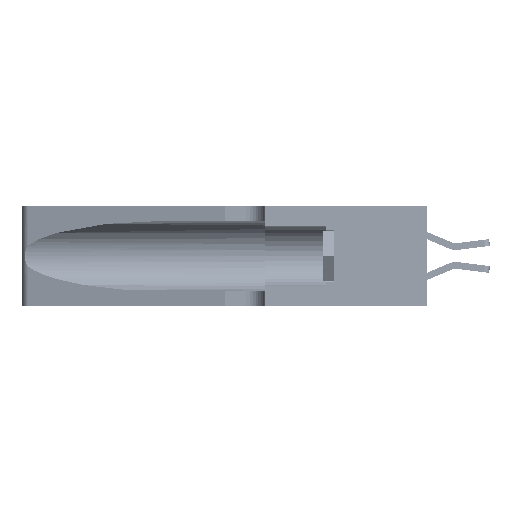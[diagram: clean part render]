
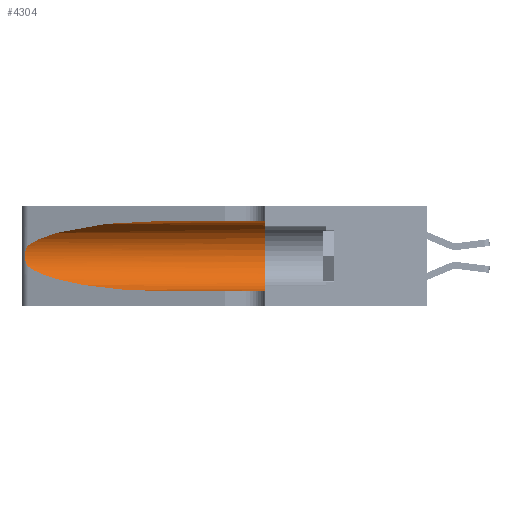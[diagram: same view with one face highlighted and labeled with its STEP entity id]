
A CAD part, left-side view. The second image highlights one B-rep face of the part: STEP entity #4304.
In plain terms, the highlighted cylindrical face has radius 3.308 mm (diameter 6.617 mm), a partial arc.
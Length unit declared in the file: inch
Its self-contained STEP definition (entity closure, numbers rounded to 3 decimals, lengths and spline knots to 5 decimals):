
#929 = ORIENTED_EDGE ( 'NONE', *, *, #17783, .T. ) ;
#1573 = B_SPLINE_CURVE_WITH_KNOTS ( 'NONE', 3,
 ( #2496, #9038, #37356, #37505, #5739, #18394, #12480, #27633, #30977, #40392, #37071, #21547, #21409, #21273 ),
 .UNSPECIFIED., .F., .F.,
 ( 4, 2, 2, 2, 2, 2, 4 ),
 ( 0., 0.00027, 0.00053, 0.00107, 0.0016, 0.00187, 0.00214 ),
 .UNSPECIFIED. ) ;
#1955 = CARTESIAN_POINT ( 'NONE',  ( 0.1305, 0.35, 0.31525 ) ) ;
#2175 = CARTESIAN_POINT ( 'NONE',  ( 0.1305, 0.35, 0.185 ) ) ;
#2311 = CARTESIAN_POINT ( 'NONE',  ( 0.1305, 1.61858, 0.05475 ) ) ;
#2496 = CARTESIAN_POINT ( 'NONE',  ( 0.25487, 1.22718, 0.22369 ) ) ;
#2839 = CARTESIAN_POINT ( 'NONE',  ( 0.25487, 1.22718, 0.22369 ) ) ;
#4304 = ADVANCED_FACE ( 'NONE', ( #5860 ), #30027, .F. ) ;
#5739 = CARTESIAN_POINT ( 'NONE',  ( 0.25854, 1.2359, 0.20912 ) ) ;
#5860 = FACE_OUTER_BOUND ( 'NONE', #28260, .T. ) ;
#6360 = CARTESIAN_POINT ( 'NONE',  ( 0.2373, 1.15595, 0.28018 ) ) ;
#6458 = EDGE_CURVE ( 'NONE', #25849, #38129, #1573, .T. ) ;
#6865 = VERTEX_POINT ( 'NONE', #19688 ) ;
#7002 =( BOUNDED_CURVE ( )  B_SPLINE_CURVE ( 3, ( #29686, #35947, #21110, #39104 ),
 .UNSPECIFIED., .F., .T. ) 
 B_SPLINE_CURVE_WITH_KNOTS ( ( 4, 4 ),
 ( 3.44316, 4.71239 ),
 .UNSPECIFIED. ) 
 CURVE ( )  GEOMETRIC_REPRESENTATION_ITEM ( )  RATIONAL_B_SPLINE_CURVE ( ( 1., 0.87, 0.87, 1. ) ) 
 REPRESENTATION_ITEM ( '' )  );
#7755 = ORIENTED_EDGE ( 'NONE', *, *, #6458, .T. ) ;
#8426 = DIRECTION ( 'NONE',  ( 0., 0., 1. ) ) ;
#8849 = ORIENTED_EDGE ( 'NONE', *, *, #15151, .F. ) ;
#9038 = CARTESIAN_POINT ( 'NONE',  ( 0.25555, 1.22994, 0.2215 ) ) ;
#9274 = ORIENTED_EDGE ( 'NONE', *, *, #15804, .T. ) ;
#9495 = CARTESIAN_POINT ( 'NONE',  ( 0.25487, 1.22718, 0.22369 ) ) ;
#11126 = VERTEX_POINT ( 'NONE', #14381 ) ;
#11443 = AXIS2_PLACEMENT_3D ( 'NONE', #15407, #16076, #38594 ) ;
#11746 = DIRECTION ( 'NONE',  ( 0., -1., 0. ) ) ;
#12480 = CARTESIAN_POINT ( 'NONE',  ( 0.26075, 1.23896, 0.19203 ) ) ;
#14381 = CARTESIAN_POINT ( 'NONE',  ( 0.1305, 0.72297, 0.05475 ) ) ;
#14624 = DIRECTION ( 'NONE',  ( 0., 1., 0. ) ) ;
#14843 = LINE ( 'NONE', #2311, #28603 ) ;
#15036 = CARTESIAN_POINT ( 'NONE',  ( 0.18966, 0.96281, 0.31525 ) ) ;
#15151 = EDGE_CURVE ( 'NONE', #18661, #6865, #29658, .T. ) ;
#15407 = CARTESIAN_POINT ( 'NONE',  ( 0.1305, 1.61858, 0.185 ) ) ;
#15804 = EDGE_CURVE ( 'NONE', #11126, #6865, #14843, .T. ) ;
#16076 = DIRECTION ( 'NONE',  ( 0., -1., 0. ) ) ;
#16973 = VERTEX_POINT ( 'NONE', #21373 ) ;
#17783 = EDGE_CURVE ( 'NONE', #38129, #11126, #7002, .T. ) ;
#18085 = ORIENTED_EDGE ( 'NONE', *, *, #18715, .T. ) ;
#18293 = LINE ( 'NONE', #31144, #34518 ) ;
#18394 = CARTESIAN_POINT ( 'NONE',  ( 0.26018, 1.23835, 0.19895 ) ) ;
#18661 = VERTEX_POINT ( 'NONE', #1955 ) ;
#18715 = EDGE_CURVE ( 'NONE', #16973, #25849, #19114, .T. ) ;
#19114 =( BOUNDED_CURVE ( )  B_SPLINE_CURVE ( 3, ( #24544, #15036, #6360, #9495 ),
 .UNSPECIFIED., .F., .F. ) 
 B_SPLINE_CURVE_WITH_KNOTS ( ( 4, 4 ),
 ( 1.5708, 2.84003 ),
 .UNSPECIFIED. ) 
 CURVE ( )  GEOMETRIC_REPRESENTATION_ITEM ( )  RATIONAL_B_SPLINE_CURVE ( ( 1., 0.87, 0.87, 1. ) ) 
 REPRESENTATION_ITEM ( '' )  );
#19593 = ORIENTED_EDGE ( 'NONE', *, *, #20591, .F. ) ;
#19688 = CARTESIAN_POINT ( 'NONE',  ( 0.1305, 0.35, 0.05475 ) ) ;
#20591 = EDGE_CURVE ( 'NONE', #16973, #18661, #18293, .T. ) ;
#21110 = CARTESIAN_POINT ( 'NONE',  ( 0.18966, 0.96281, 0.05475 ) ) ;
#21273 = CARTESIAN_POINT ( 'NONE',  ( 0.25487, 1.22718, 0.14631 ) ) ;
#21373 = CARTESIAN_POINT ( 'NONE',  ( 0.1305, 0.72297, 0.31525 ) ) ;
#21409 = CARTESIAN_POINT ( 'NONE',  ( 0.25555, 1.22993, 0.14849 ) ) ;
#21547 = CARTESIAN_POINT ( 'NONE',  ( 0.25639, 1.23186, 0.15144 ) ) ;
#24544 = CARTESIAN_POINT ( 'NONE',  ( 0.1305, 0.72297, 0.31525 ) ) ;
#25849 = VERTEX_POINT ( 'NONE', #2839 ) ;
#27633 = CARTESIAN_POINT ( 'NONE',  ( 0.26075, 1.23896, 0.178 ) ) ;
#28082 = DIRECTION ( 'NONE',  ( 0., -1., 0. ) ) ;
#28116 = CARTESIAN_POINT ( 'NONE',  ( 0.25487, 1.22718, 0.14631 ) ) ;
#28260 = EDGE_LOOP ( 'NONE', ( #18085, #7755, #929, #9274, #8849, #19593 ) ) ;
#28603 = VECTOR ( 'NONE', #11746, 39.37008 ) ;
#29658 = CIRCLE ( 'NONE', #30846, 0.13025 ) ;
#29686 = CARTESIAN_POINT ( 'NONE',  ( 0.25487, 1.22718, 0.14631 ) ) ;
#30027 = CYLINDRICAL_SURFACE ( 'NONE', #11443, 0.13025 ) ;
#30846 = AXIS2_PLACEMENT_3D ( 'NONE', #2175, #14624, #8426 ) ;
#30977 = CARTESIAN_POINT ( 'NONE',  ( 0.26017, 1.23833, 0.17102 ) ) ;
#31144 = CARTESIAN_POINT ( 'NONE',  ( 0.1305, 1.61858, 0.31525 ) ) ;
#34518 = VECTOR ( 'NONE', #28082, 39.37008 ) ;
#35947 = CARTESIAN_POINT ( 'NONE',  ( 0.2373, 1.15595, 0.08982 ) ) ;
#37071 = CARTESIAN_POINT ( 'NONE',  ( 0.25789, 1.23486, 0.15765 ) ) ;
#37356 = CARTESIAN_POINT ( 'NONE',  ( 0.25639, 1.23184, 0.21858 ) ) ;
#37505 = CARTESIAN_POINT ( 'NONE',  ( 0.25787, 1.23484, 0.2124 ) ) ;
#38129 = VERTEX_POINT ( 'NONE', #28116 ) ;
#38594 = DIRECTION ( 'NONE',  ( 0., 0., -1. ) ) ;
#39104 = CARTESIAN_POINT ( 'NONE',  ( 0.1305, 0.72297, 0.05475 ) ) ;
#40392 = CARTESIAN_POINT ( 'NONE',  ( 0.25856, 1.23593, 0.16098 ) ) ;
